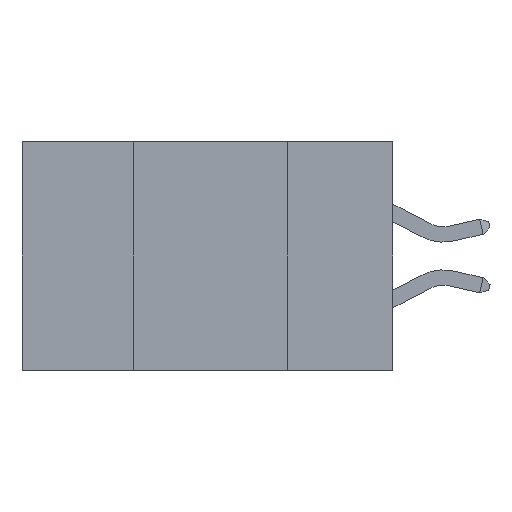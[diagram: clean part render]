
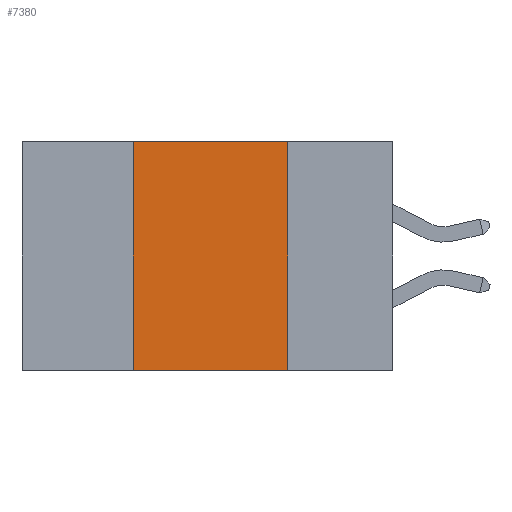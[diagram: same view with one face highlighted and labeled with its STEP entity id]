
A CAD part, left-side view. The second image highlights one B-rep face of the part: STEP entity #7380.
In plain terms, the highlighted planar face has unit normal (-1, 0, 0).
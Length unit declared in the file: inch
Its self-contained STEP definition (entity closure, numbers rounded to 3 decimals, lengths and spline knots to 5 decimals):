
#159 = DIRECTION ( 'NONE',  ( 0., 0., -1. ) ) ;
#165 = DIRECTION ( 'NONE',  ( 0., -1., 0. ) ) ;
#398 = CARTESIAN_POINT ( 'NONE',  ( 0., 0.17, 0. ) ) ;
#638 = AXIS2_PLACEMENT_3D ( 'NONE', #4076, #4658, #12064 ) ;
#1826 = LINE ( 'NONE', #17496, #16980 ) ;
#2829 = VERTEX_POINT ( 'NONE', #7472 ) ;
#3552 = FACE_OUTER_BOUND ( 'NONE', #15930, .T. ) ;
#4076 = CARTESIAN_POINT ( 'NONE',  ( 0., 0.6, 0. ) ) ;
#4658 = DIRECTION ( 'NONE',  ( 1., 0., 0. ) ) ;
#5767 = ORIENTED_EDGE ( 'NONE', *, *, #18984, .F. ) ;
#6807 = VECTOR ( 'NONE', #159, 39.37008 ) ;
#7380 = ADVANCED_FACE ( 'NONE', ( #3552 ), #7576, .F. ) ;
#7472 = CARTESIAN_POINT ( 'NONE',  ( 0., 0.42, 0. ) ) ;
#7576 = PLANE ( 'NONE',  #638 ) ;
#8574 = CARTESIAN_POINT ( 'NONE',  ( 0., 0.42, 0. ) ) ;
#8716 = DIRECTION ( 'NONE',  ( 0., 0., 1. ) ) ;
#10197 = EDGE_CURVE ( 'NONE', #13396, #18426, #1826, .T. ) ;
#10433 = LINE ( 'NONE', #11976, #6807 ) ;
#11741 = LINE ( 'NONE', #18793, #16771 ) ;
#11976 = CARTESIAN_POINT ( 'NONE',  ( 0., 0.17, 0. ) ) ;
#12064 = DIRECTION ( 'NONE',  ( 0., 0., -1. ) ) ;
#12672 = EDGE_CURVE ( 'NONE', #13396, #2829, #18837, .T. ) ;
#13310 = CARTESIAN_POINT ( 'NONE',  ( 0., 0.42, -0.37 ) ) ;
#13396 = VERTEX_POINT ( 'NONE', #13310 ) ;
#14311 = DIRECTION ( 'NONE',  ( 0., -1., 0. ) ) ;
#15050 = VERTEX_POINT ( 'NONE', #398 ) ;
#15096 = ORIENTED_EDGE ( 'NONE', *, *, #12672, .F. ) ;
#15930 = EDGE_LOOP ( 'NONE', ( #16778, #5767, #15096, #16849 ) ) ;
#16065 = EDGE_CURVE ( 'NONE', #15050, #18426, #10433, .T. ) ;
#16771 = VECTOR ( 'NONE', #14311, 39.37008 ) ;
#16778 = ORIENTED_EDGE ( 'NONE', *, *, #16065, .F. ) ;
#16849 = ORIENTED_EDGE ( 'NONE', *, *, #10197, .T. ) ;
#16980 = VECTOR ( 'NONE', #165, 39.37008 ) ;
#17131 = CARTESIAN_POINT ( 'NONE',  ( 0., 0.17, -0.37 ) ) ;
#17213 = VECTOR ( 'NONE', #8716, 39.37008 ) ;
#17496 = CARTESIAN_POINT ( 'NONE',  ( 0., 0.6, -0.37 ) ) ;
#18426 = VERTEX_POINT ( 'NONE', #17131 ) ;
#18793 = CARTESIAN_POINT ( 'NONE',  ( 0., 0.6, 0. ) ) ;
#18837 = LINE ( 'NONE', #8574, #17213 ) ;
#18984 = EDGE_CURVE ( 'NONE', #2829, #15050, #11741, .T. ) ;
